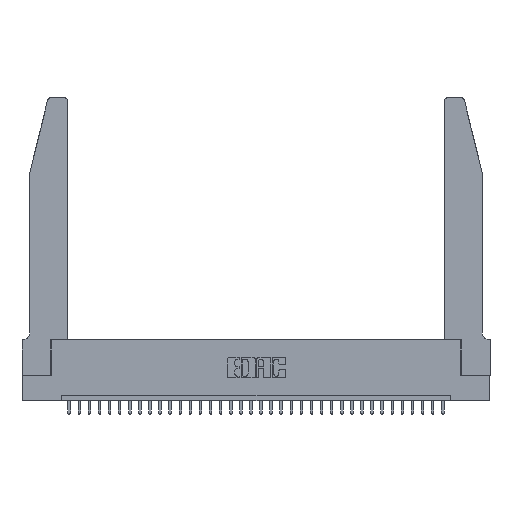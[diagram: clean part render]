
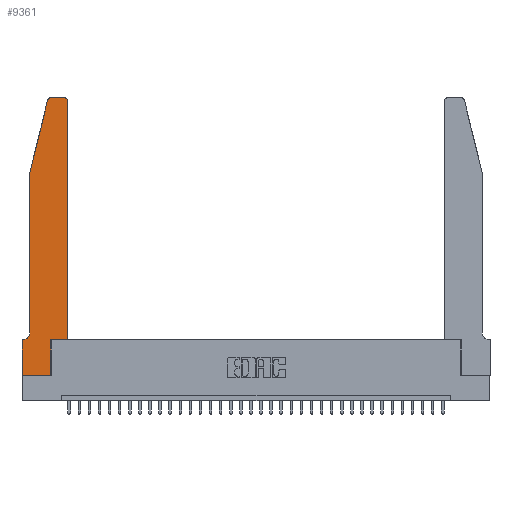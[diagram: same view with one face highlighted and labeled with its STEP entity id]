
A CAD part, top view. The second image highlights one B-rep face of the part: STEP entity #9361.
In plain terms, the highlighted planar face has unit normal (0, 0, 1).
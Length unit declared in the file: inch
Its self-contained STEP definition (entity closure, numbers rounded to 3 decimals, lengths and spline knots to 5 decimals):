
#89 = DIRECTION ( 'NONE',  ( 0., 1., 0. ) ) ;
#207 = LINE ( 'NONE', #15092, #7145 ) ;
#449 = VECTOR ( 'NONE', #25811, 39.37008 ) ;
#785 = VECTOR ( 'NONE', #89, 39.37008 ) ;
#1241 = EDGE_LOOP ( 'NONE', ( #31812, #3394, #10863, #28068, #21069, #20967, #19009, #25119, #12509, #9920, #16229, #17869 ) ) ;
#1865 = VERTEX_POINT ( 'NONE', #11686 ) ;
#2396 = VERTEX_POINT ( 'NONE', #32250 ) ;
#2440 = CARTESIAN_POINT ( 'NONE',  ( 0., 0.35, 0.37 ) ) ;
#2731 = CARTESIAN_POINT ( 'NONE',  ( 0., 0., 0.37 ) ) ;
#2740 = EDGE_CURVE ( 'NONE', #8129, #28025, #207, .T. ) ;
#3222 = LINE ( 'NONE', #13254, #785 ) ;
#3394 = ORIENTED_EDGE ( 'NONE', *, *, #17676, .T. ) ;
#4048 = CARTESIAN_POINT ( 'NONE',  ( 0.25487, 2.72718, 0.37 ) ) ;
#4575 = VERTEX_POINT ( 'NONE', #2440 ) ;
#4673 = FACE_OUTER_BOUND ( 'NONE', #1241, .T. ) ;
#5896 = EDGE_CURVE ( 'NONE', #11498, #19681, #7378, .T. ) ;
#6319 = DIRECTION ( 'NONE',  ( 1., 0., 0. ) ) ;
#7145 = VECTOR ( 'NONE', #33500, 39.37008 ) ;
#7208 = VERTEX_POINT ( 'NONE', #24338 ) ;
#7378 = LINE ( 'NONE', #23190, #449 ) ;
#7381 = DIRECTION ( 'NONE',  ( 1., 0., 0. ) ) ;
#7863 = EDGE_CURVE ( 'NONE', #4575, #18473, #19142, .T. ) ;
#7930 = AXIS2_PLACEMENT_3D ( 'NONE', #30978, #15535, #23501 ) ;
#8129 = VERTEX_POINT ( 'NONE', #26508 ) ;
#8145 = LINE ( 'NONE', #17582, #27823 ) ;
#9361 = ADVANCED_FACE ( 'NONE', ( #4673 ), #20587, .T. ) ;
#9494 = CARTESIAN_POINT ( 'NONE',  ( 0., 0., 0.37 ) ) ;
#9920 = ORIENTED_EDGE ( 'NONE', *, *, #28740, .T. ) ;
#10539 = VECTOR ( 'NONE', #27880, 39.37008 ) ;
#10818 = AXIS2_PLACEMENT_3D ( 'NONE', #23063, #12460, #7381 ) ;
#10863 = ORIENTED_EDGE ( 'NONE', *, *, #5896, .T. ) ;
#11498 = VERTEX_POINT ( 'NONE', #4048 ) ;
#11686 = CARTESIAN_POINT ( 'NONE',  ( 0.2865, 0.35, 0.37 ) ) ;
#12190 = VECTOR ( 'NONE', #20729, 39.37008 ) ;
#12460 = DIRECTION ( 'NONE',  ( 0., 0., 1. ) ) ;
#12509 = ORIENTED_EDGE ( 'NONE', *, *, #25391, .T. ) ;
#12681 = DIRECTION ( 'NONE',  ( -1., 0., 0. ) ) ;
#13254 = CARTESIAN_POINT ( 'NONE',  ( 0.2865, 0.35, 0.37 ) ) ;
#13625 = EDGE_CURVE ( 'NONE', #28025, #21530, #29092, .T. ) ;
#13761 = DIRECTION ( 'NONE',  ( -1., 0., 0. ) ) ;
#14254 = DIRECTION ( 'NONE',  ( 0., 0., 1. ) ) ;
#15092 = CARTESIAN_POINT ( 'NONE',  ( 0.4505, 0.35, 0.37 ) ) ;
#15535 = DIRECTION ( 'NONE',  ( 0., 0., -1. ) ) ;
#16229 = ORIENTED_EDGE ( 'NONE', *, *, #2740, .T. ) ;
#16514 = CARTESIAN_POINT ( 'NONE',  ( 0.4505, 2.72, 0.37 ) ) ;
#17582 = CARTESIAN_POINT ( 'NONE',  ( 0., 0., 0.37 ) ) ;
#17676 = EDGE_CURVE ( 'NONE', #2396, #11498, #31861, .T. ) ;
#17869 = ORIENTED_EDGE ( 'NONE', *, *, #13625, .T. ) ;
#18311 = LINE ( 'NONE', #22178, #10539 ) ;
#18378 = EDGE_CURVE ( 'NONE', #19681, #22780, #18311, .T. ) ;
#18473 = VERTEX_POINT ( 'NONE', #9494 ) ;
#18763 = CARTESIAN_POINT ( 'NONE',  ( 0.0055, 0.35, 0.37 ) ) ;
#18870 = VECTOR ( 'NONE', #13761, 39.37008 ) ;
#19007 = LINE ( 'NONE', #20362, #20251 ) ;
#19009 = ORIENTED_EDGE ( 'NONE', *, *, #7863, .T. ) ;
#19142 = LINE ( 'NONE', #2731, #12190 ) ;
#19681 = VERTEX_POINT ( 'NONE', #23181 ) ;
#20251 = VECTOR ( 'NONE', #12681, 39.37008 ) ;
#20275 = CARTESIAN_POINT ( 'NONE',  ( 0.0755, 0.42, 0.37 ) ) ;
#20362 = CARTESIAN_POINT ( 'NONE',  ( 0.2605, 2.75, 0.37 ) ) ;
#20566 = DIRECTION ( 'NONE',  ( 1., 0., 0. ) ) ;
#20587 = PLANE ( 'NONE',  #10818 ) ;
#20729 = DIRECTION ( 'NONE',  ( 0., -1., 0. ) ) ;
#20967 = ORIENTED_EDGE ( 'NONE', *, *, #33087, .T. ) ;
#21069 = ORIENTED_EDGE ( 'NONE', *, *, #32168, .T. ) ;
#21530 = VERTEX_POINT ( 'NONE', #24188 ) ;
#21688 = AXIS2_PLACEMENT_3D ( 'NONE', #27266, #22024, #21797 ) ;
#21797 = DIRECTION ( 'NONE',  ( 1., 0., 0. ) ) ;
#22024 = DIRECTION ( 'NONE',  ( 0., 0., 1. ) ) ;
#22178 = CARTESIAN_POINT ( 'NONE',  ( 0.0755, 2., 0.37 ) ) ;
#22780 = VERTEX_POINT ( 'NONE', #20275 ) ;
#23063 = CARTESIAN_POINT ( 'NONE',  ( 0., 0.35, 0.37 ) ) ;
#23181 = CARTESIAN_POINT ( 'NONE',  ( 0.0755, 2., 0.37 ) ) ;
#23190 = CARTESIAN_POINT ( 'NONE',  ( 0.0755, 2., 0.37 ) ) ;
#23501 = DIRECTION ( 'NONE',  ( -1., 0., 0. ) ) ;
#23794 = VERTEX_POINT ( 'NONE', #18763 ) ;
#23916 = CARTESIAN_POINT ( 'NONE',  ( 0.0755, 0.35, 0.37 ) ) ;
#24188 = CARTESIAN_POINT ( 'NONE',  ( 0.4205, 2.75, 0.37 ) ) ;
#24338 = CARTESIAN_POINT ( 'NONE',  ( 0.2865, 0., 0.37 ) ) ;
#24785 = EDGE_CURVE ( 'NONE', #18473, #7208, #8145, .T. ) ;
#24817 = DIRECTION ( 'NONE',  ( 1., 0., 0. ) ) ;
#25119 = ORIENTED_EDGE ( 'NONE', *, *, #24785, .T. ) ;
#25391 = EDGE_CURVE ( 'NONE', #7208, #1865, #3222, .T. ) ;
#25811 = DIRECTION ( 'NONE',  ( -0.239, -0.971, 0. ) ) ;
#26508 = CARTESIAN_POINT ( 'NONE',  ( 0.4505, 0.35, 0.37 ) ) ;
#27266 = CARTESIAN_POINT ( 'NONE',  ( 0.284, 2.72, 0.37 ) ) ;
#27489 = CIRCLE ( 'NONE', #7930, 0.07 ) ;
#27823 = VECTOR ( 'NONE', #20566, 39.37008 ) ;
#27880 = DIRECTION ( 'NONE',  ( 0., -1., 0. ) ) ;
#28025 = VERTEX_POINT ( 'NONE', #16514 ) ;
#28068 = ORIENTED_EDGE ( 'NONE', *, *, #18378, .T. ) ;
#28740 = EDGE_CURVE ( 'NONE', #1865, #8129, #30012, .T. ) ;
#28794 = VECTOR ( 'NONE', #24817, 39.37008 ) ;
#29092 = CIRCLE ( 'NONE', #33493, 0.03 ) ;
#29806 = CARTESIAN_POINT ( 'NONE',  ( 0.4205, 2.72, 0.37 ) ) ;
#30012 = LINE ( 'NONE', #32489, #28794 ) ;
#30978 = CARTESIAN_POINT ( 'NONE',  ( 0.0055, 0.42, 0.37 ) ) ;
#31458 = EDGE_CURVE ( 'NONE', #21530, #2396, #19007, .T. ) ;
#31812 = ORIENTED_EDGE ( 'NONE', *, *, #31458, .T. ) ;
#31861 = CIRCLE ( 'NONE', #21688, 0.03 ) ;
#32168 = EDGE_CURVE ( 'NONE', #22780, #23794, #27489, .T. ) ;
#32250 = CARTESIAN_POINT ( 'NONE',  ( 0.284, 2.75, 0.37 ) ) ;
#32489 = CARTESIAN_POINT ( 'NONE',  ( 0.4505, 0.35, 0.37 ) ) ;
#32809 = LINE ( 'NONE', #23916, #18870 ) ;
#33087 = EDGE_CURVE ( 'NONE', #23794, #4575, #32809, .T. ) ;
#33493 = AXIS2_PLACEMENT_3D ( 'NONE', #29806, #14254, #6319 ) ;
#33500 = DIRECTION ( 'NONE',  ( 0., 1., 0. ) ) ;
